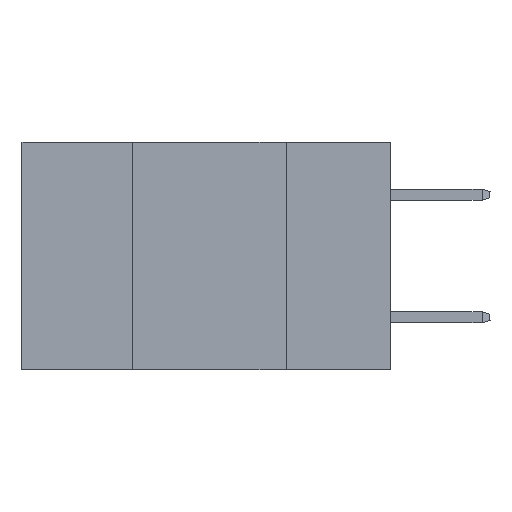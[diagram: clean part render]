
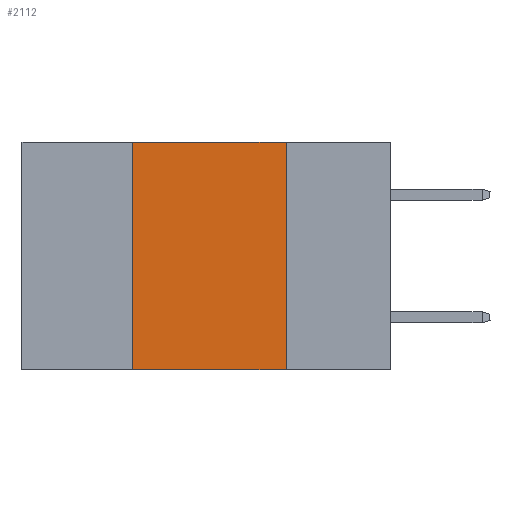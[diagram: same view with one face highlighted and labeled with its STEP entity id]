
A CAD part, left-side view. The second image highlights one B-rep face of the part: STEP entity #2112.
In plain terms, the highlighted planar face has unit normal (-1, 0, 0).
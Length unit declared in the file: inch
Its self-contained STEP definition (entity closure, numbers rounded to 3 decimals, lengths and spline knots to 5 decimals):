
#915 = CARTESIAN_POINT ( 'NONE',  ( 0., 0.6, 0. ) ) ;
#1561 = VECTOR ( 'NONE', #24042, 39.37008 ) ;
#2112 = ADVANCED_FACE ( 'NONE', ( #16940 ), #2405, .F. ) ;
#2116 = LINE ( 'NONE', #27424, #15823 ) ;
#2300 = CARTESIAN_POINT ( 'NONE',  ( 0., 0.6, 0. ) ) ;
#2405 = PLANE ( 'NONE',  #27275 ) ;
#4061 = CARTESIAN_POINT ( 'NONE',  ( 0., 0.42, -0.37 ) ) ;
#4606 = EDGE_LOOP ( 'NONE', ( #15634, #20177, #19594, #29552 ) ) ;
#7994 = CARTESIAN_POINT ( 'NONE',  ( 0., 0.17, -0.37 ) ) ;
#8245 = VERTEX_POINT ( 'NONE', #7994 ) ;
#8875 = DIRECTION ( 'NONE',  ( 0., 0., -1. ) ) ;
#9071 = CARTESIAN_POINT ( 'NONE',  ( 0., 0.17, 0. ) ) ;
#9310 = DIRECTION ( 'NONE',  ( 0., 0., -1. ) ) ;
#9312 = CARTESIAN_POINT ( 'NONE',  ( 0., 0.6, -0.37 ) ) ;
#11139 = VECTOR ( 'NONE', #16298, 39.37008 ) ;
#12049 = EDGE_CURVE ( 'NONE', #13848, #18132, #18141, .T. ) ;
#13375 = DIRECTION ( 'NONE',  ( 0., 0., 1. ) ) ;
#13848 = VERTEX_POINT ( 'NONE', #27018 ) ;
#14615 = CARTESIAN_POINT ( 'NONE',  ( 0., 0.17, 0. ) ) ;
#14677 = EDGE_CURVE ( 'NONE', #15778, #8245, #15489, .T. ) ;
#15489 = LINE ( 'NONE', #9312, #11139 ) ;
#15634 = ORIENTED_EDGE ( 'NONE', *, *, #17091, .F. ) ;
#15778 = VERTEX_POINT ( 'NONE', #4061 ) ;
#15823 = VECTOR ( 'NONE', #13375, 39.37008 ) ;
#16298 = DIRECTION ( 'NONE',  ( 0., -1., 0. ) ) ;
#16940 = FACE_OUTER_BOUND ( 'NONE', #4606, .T. ) ;
#17091 = EDGE_CURVE ( 'NONE', #18132, #8245, #21772, .T. ) ;
#18132 = VERTEX_POINT ( 'NONE', #14615 ) ;
#18141 = LINE ( 'NONE', #915, #1561 ) ;
#19594 = ORIENTED_EDGE ( 'NONE', *, *, #21623, .F. ) ;
#20177 = ORIENTED_EDGE ( 'NONE', *, *, #12049, .F. ) ;
#21623 = EDGE_CURVE ( 'NONE', #15778, #13848, #2116, .T. ) ;
#21772 = LINE ( 'NONE', #9071, #24649 ) ;
#24042 = DIRECTION ( 'NONE',  ( 0., -1., 0. ) ) ;
#24649 = VECTOR ( 'NONE', #8875, 39.37008 ) ;
#27018 = CARTESIAN_POINT ( 'NONE',  ( 0., 0.42, 0. ) ) ;
#27275 = AXIS2_PLACEMENT_3D ( 'NONE', #2300, #27389, #9310 ) ;
#27389 = DIRECTION ( 'NONE',  ( 1., 0., 0. ) ) ;
#27424 = CARTESIAN_POINT ( 'NONE',  ( 0., 0.42, 0. ) ) ;
#29552 = ORIENTED_EDGE ( 'NONE', *, *, #14677, .T. ) ;
